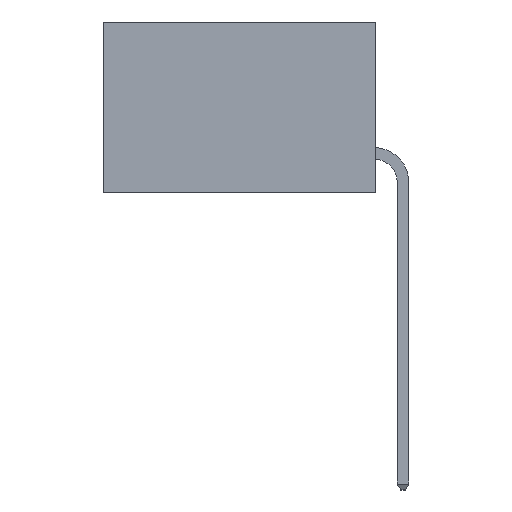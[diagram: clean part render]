
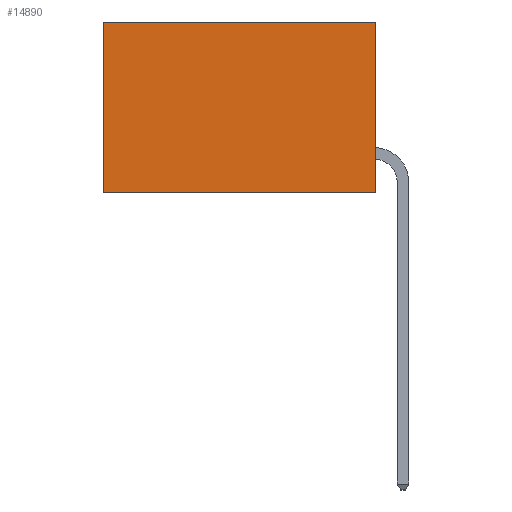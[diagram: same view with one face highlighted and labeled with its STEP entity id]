
A CAD part, left-side view. The second image highlights one B-rep face of the part: STEP entity #14890.
In plain terms, the highlighted planar face has unit normal (-1, 0, 0).
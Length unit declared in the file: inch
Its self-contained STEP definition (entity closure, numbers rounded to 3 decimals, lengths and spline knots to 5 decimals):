
#397 = FACE_OUTER_BOUND ( 'NONE', #19181, .T. ) ;
#1397 = ORIENTED_EDGE ( 'NONE', *, *, #8205, .F. ) ;
#1846 = VECTOR ( 'NONE', #9474, 39.37008 ) ;
#1856 = CARTESIAN_POINT ( 'NONE',  ( 0.277, 0., -0.37 ) ) ;
#2992 = VERTEX_POINT ( 'NONE', #22955 ) ;
#3113 = VERTEX_POINT ( 'NONE', #22119 ) ;
#4813 = DIRECTION ( 'NONE',  ( 0., 0., -1. ) ) ;
#7565 = LINE ( 'NONE', #26520, #1846 ) ;
#7608 = AXIS2_PLACEMENT_3D ( 'NONE', #19912, #22060, #9196 ) ;
#8205 = EDGE_CURVE ( 'NONE', #23948, #9837, #7565, .T. ) ;
#8214 = ORIENTED_EDGE ( 'NONE', *, *, #20766, .T. ) ;
#8475 = LINE ( 'NONE', #9989, #19887 ) ;
#9196 = DIRECTION ( 'NONE',  ( 0., 0., -1. ) ) ;
#9474 = DIRECTION ( 'NONE',  ( 0., 1., 0. ) ) ;
#9837 = VERTEX_POINT ( 'NONE', #15248 ) ;
#9989 = CARTESIAN_POINT ( 'NONE',  ( 0.277, 0., -0.37 ) ) ;
#11191 = LINE ( 'NONE', #19848, #27572 ) ;
#11216 = LINE ( 'NONE', #25528, #21285 ) ;
#13494 = ORIENTED_EDGE ( 'NONE', *, *, #14761, .F. ) ;
#14761 = EDGE_CURVE ( 'NONE', #3113, #23948, #8475, .T. ) ;
#14890 = ADVANCED_FACE ( 'NONE', ( #397 ), #17743, .F. ) ;
#15248 = CARTESIAN_POINT ( 'NONE',  ( 0.277, 0.59, -0.37 ) ) ;
#17743 = PLANE ( 'NONE',  #7608 ) ;
#19181 = EDGE_LOOP ( 'NONE', ( #22037, #1397, #13494, #8214 ) ) ;
#19848 = CARTESIAN_POINT ( 'NONE',  ( 0.277, 0.59, -0.37 ) ) ;
#19887 = VECTOR ( 'NONE', #24996, 39.37008 ) ;
#19912 = CARTESIAN_POINT ( 'NONE',  ( 0.277, 0., -0.37 ) ) ;
#20766 = EDGE_CURVE ( 'NONE', #3113, #2992, #11216, .T. ) ;
#21201 = EDGE_CURVE ( 'NONE', #2992, #9837, #11191, .T. ) ;
#21221 = DIRECTION ( 'NONE',  ( 0., 1., 0. ) ) ;
#21285 = VECTOR ( 'NONE', #21221, 39.37008 ) ;
#22037 = ORIENTED_EDGE ( 'NONE', *, *, #21201, .T. ) ;
#22060 = DIRECTION ( 'NONE',  ( 1., 0., 0. ) ) ;
#22119 = CARTESIAN_POINT ( 'NONE',  ( 0.277, 0., 0. ) ) ;
#22955 = CARTESIAN_POINT ( 'NONE',  ( 0.277, 0.59, 0. ) ) ;
#23948 = VERTEX_POINT ( 'NONE', #1856 ) ;
#24996 = DIRECTION ( 'NONE',  ( 0., 0., -1. ) ) ;
#25528 = CARTESIAN_POINT ( 'NONE',  ( 0.277, 0., 0. ) ) ;
#26520 = CARTESIAN_POINT ( 'NONE',  ( 0.277, 0., -0.37 ) ) ;
#27572 = VECTOR ( 'NONE', #4813, 39.37008 ) ;
